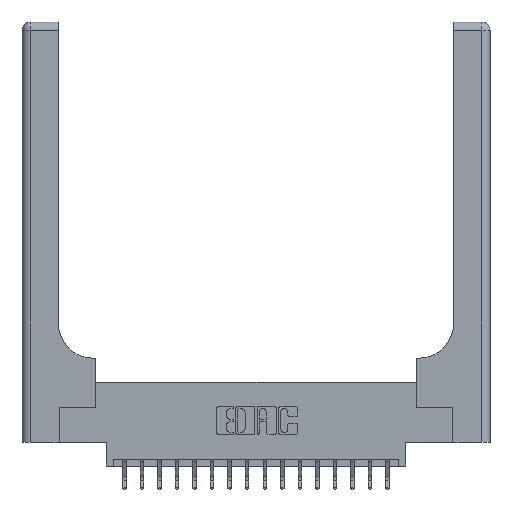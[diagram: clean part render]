
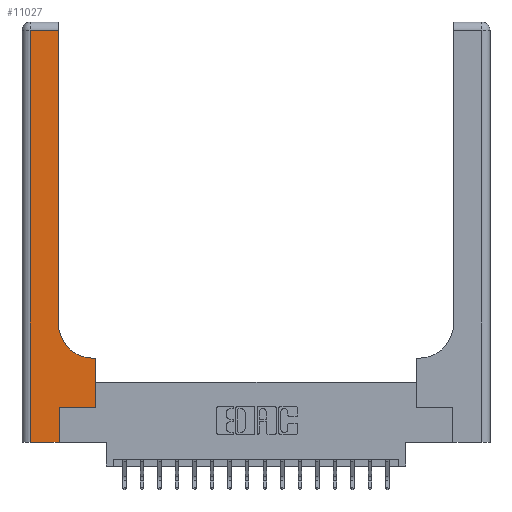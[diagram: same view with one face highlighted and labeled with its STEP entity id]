
A CAD part, top view. The second image highlights one B-rep face of the part: STEP entity #11027.
In plain terms, the highlighted planar face has unit normal (0, 0, 1).
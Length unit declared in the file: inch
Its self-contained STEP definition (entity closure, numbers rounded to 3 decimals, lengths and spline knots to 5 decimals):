
#543 = CARTESIAN_POINT ( 'NONE',  ( 0.265, 0., 0.37 ) ) ;
#652 = DIRECTION ( 'NONE',  ( 1., 0., 0. ) ) ;
#795 = EDGE_CURVE ( 'NONE', #13832, #4599, #16428, .T. ) ;
#1325 = CARTESIAN_POINT ( 'NONE',  ( 0., 2.94, 0.37 ) ) ;
#1560 = ORIENTED_EDGE ( 'NONE', *, *, #3828, .T. ) ;
#1639 = DIRECTION ( 'NONE',  ( -1., 0., 0. ) ) ;
#2111 = VERTEX_POINT ( 'NONE', #13899 ) ;
#2468 = EDGE_LOOP ( 'NONE', ( #9295, #8374, #2970, #6052, #1560, #12231, #6233, #3898, #14841 ) ) ;
#2481 = VECTOR ( 'NONE', #19137, 39.37008 ) ;
#2615 = CARTESIAN_POINT ( 'NONE',  ( 0.06, 3., 0.37 ) ) ;
#2728 = EDGE_CURVE ( 'NONE', #18474, #11544, #5578, .T. ) ;
#2857 = PLANE ( 'NONE',  #19798 ) ;
#2888 = VERTEX_POINT ( 'NONE', #9011 ) ;
#2970 = ORIENTED_EDGE ( 'NONE', *, *, #795, .T. ) ;
#3003 = EDGE_CURVE ( 'NONE', #8588, #5491, #14609, .T. ) ;
#3047 = DIRECTION ( 'NONE',  ( 0., 0., -1. ) ) ;
#3494 = VECTOR ( 'NONE', #8995, 39.37008 ) ;
#3828 = EDGE_CURVE ( 'NONE', #2111, #18474, #19090, .T. ) ;
#3898 = ORIENTED_EDGE ( 'NONE', *, *, #5225, .T. ) ;
#4599 = VERTEX_POINT ( 'NONE', #17218 ) ;
#4795 = VECTOR ( 'NONE', #8008, 39.37008 ) ;
#4903 = CARTESIAN_POINT ( 'NONE',  ( 0.528, 0.25, 0.37 ) ) ;
#5225 = EDGE_CURVE ( 'NONE', #2888, #6952, #13856, .T. ) ;
#5491 = VERTEX_POINT ( 'NONE', #6401 ) ;
#5578 = LINE ( 'NONE', #13355, #17587 ) ;
#6052 = ORIENTED_EDGE ( 'NONE', *, *, #10819, .T. ) ;
#6170 = CARTESIAN_POINT ( 'NONE',  ( 0.528, 0.25, 0.37 ) ) ;
#6233 = ORIENTED_EDGE ( 'NONE', *, *, #6769, .T. ) ;
#6282 = CARTESIAN_POINT ( 'NONE',  ( 0.26, 3., 0.37 ) ) ;
#6401 = CARTESIAN_POINT ( 'NONE',  ( 0.26, 2.94, 0.37 ) ) ;
#6769 = EDGE_CURVE ( 'NONE', #11544, #2888, #11081, .T. ) ;
#6952 = VERTEX_POINT ( 'NONE', #11390 ) ;
#7502 = CARTESIAN_POINT ( 'NONE',  ( 0.26, 0.6, 0.37 ) ) ;
#7865 = VECTOR ( 'NONE', #652, 39.37008 ) ;
#8008 = DIRECTION ( 'NONE',  ( 0., 1., 0. ) ) ;
#8374 = ORIENTED_EDGE ( 'NONE', *, *, #17468, .T. ) ;
#8588 = VERTEX_POINT ( 'NONE', #10034 ) ;
#8879 = DIRECTION ( 'NONE',  ( 0., -1., 0. ) ) ;
#8995 = DIRECTION ( 'NONE',  ( -1., 0., 0. ) ) ;
#9011 = CARTESIAN_POINT ( 'NONE',  ( 0.528, 0.6, 0.37 ) ) ;
#9220 = DIRECTION ( 'NONE',  ( -1., 0., 0. ) ) ;
#9260 = DIRECTION ( 'NONE',  ( 0., 1., 0. ) ) ;
#9295 = ORIENTED_EDGE ( 'NONE', *, *, #3003, .T. ) ;
#9594 = VECTOR ( 'NONE', #1639, 39.37008 ) ;
#10034 = CARTESIAN_POINT ( 'NONE',  ( 0.26, 0.85, 0.37 ) ) ;
#10225 = DIRECTION ( 'NONE',  ( 1., 0., 0. ) ) ;
#10236 = CARTESIAN_POINT ( 'NONE',  ( 0.51, 0.85, 0.37 ) ) ;
#10745 = CARTESIAN_POINT ( 'NONE',  ( 0., 3., 0.37 ) ) ;
#10819 = EDGE_CURVE ( 'NONE', #4599, #2111, #19004, .T. ) ;
#11027 = ADVANCED_FACE ( 'NONE', ( #11970 ), #2857, .F. ) ;
#11081 = LINE ( 'NONE', #4903, #12294 ) ;
#11180 = CARTESIAN_POINT ( 'NONE',  ( 0.06, 2.94, 0.37 ) ) ;
#11243 = CIRCLE ( 'NONE', #19310, 0.25 ) ;
#11390 = CARTESIAN_POINT ( 'NONE',  ( 0.51, 0.6, 0.37 ) ) ;
#11544 = VERTEX_POINT ( 'NONE', #6170 ) ;
#11867 = DIRECTION ( 'NONE',  ( 0., 0., -1. ) ) ;
#11970 = FACE_OUTER_BOUND ( 'NONE', #2468, .T. ) ;
#12231 = ORIENTED_EDGE ( 'NONE', *, *, #2728, .T. ) ;
#12294 = VECTOR ( 'NONE', #9260, 39.37008 ) ;
#12815 = VECTOR ( 'NONE', #8879, 39.37008 ) ;
#13355 = CARTESIAN_POINT ( 'NONE',  ( 0.265, 0.25, 0.37 ) ) ;
#13832 = VERTEX_POINT ( 'NONE', #11180 ) ;
#13856 = LINE ( 'NONE', #7502, #9594 ) ;
#13899 = CARTESIAN_POINT ( 'NONE',  ( 0.265, 0., 0.37 ) ) ;
#13933 = LINE ( 'NONE', #1325, #3494 ) ;
#14036 = CARTESIAN_POINT ( 'NONE',  ( 0.265, 0.25, 0.37 ) ) ;
#14079 = CARTESIAN_POINT ( 'NONE',  ( 0., 0., 0.37 ) ) ;
#14609 = LINE ( 'NONE', #6282, #2481 ) ;
#14841 = ORIENTED_EDGE ( 'NONE', *, *, #16868, .T. ) ;
#14967 = DIRECTION ( 'NONE',  ( 1., 0., 0. ) ) ;
#16428 = LINE ( 'NONE', #2615, #12815 ) ;
#16868 = EDGE_CURVE ( 'NONE', #6952, #8588, #11243, .T. ) ;
#17218 = CARTESIAN_POINT ( 'NONE',  ( 0.06, 0., 0.37 ) ) ;
#17468 = EDGE_CURVE ( 'NONE', #5491, #13832, #13933, .T. ) ;
#17587 = VECTOR ( 'NONE', #10225, 39.37008 ) ;
#18474 = VERTEX_POINT ( 'NONE', #14036 ) ;
#19004 = LINE ( 'NONE', #14079, #7865 ) ;
#19090 = LINE ( 'NONE', #543, #4795 ) ;
#19137 = DIRECTION ( 'NONE',  ( 0., 1., 0. ) ) ;
#19310 = AXIS2_PLACEMENT_3D ( 'NONE', #10236, #11867, #14967 ) ;
#19798 = AXIS2_PLACEMENT_3D ( 'NONE', #10745, #3047, #9220 ) ;
